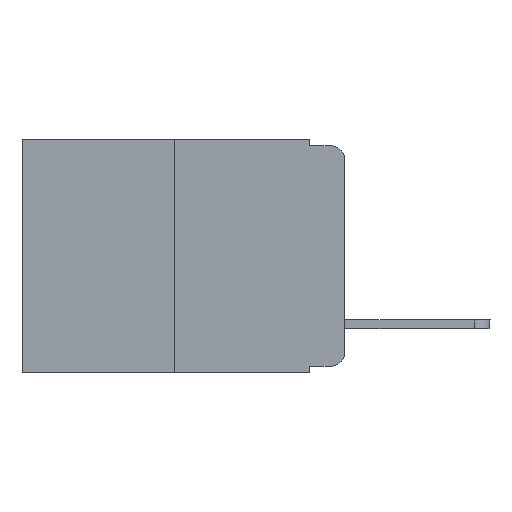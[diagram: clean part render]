
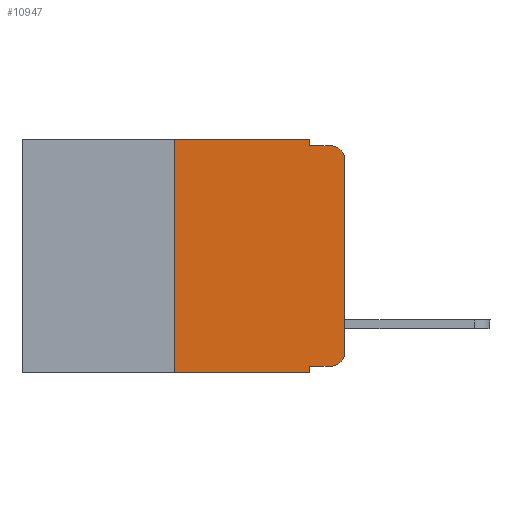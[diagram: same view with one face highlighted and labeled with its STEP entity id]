
A CAD part, left-side view. The second image highlights one B-rep face of the part: STEP entity #10947.
In plain terms, the highlighted planar face has unit normal (-1, 0, 0).
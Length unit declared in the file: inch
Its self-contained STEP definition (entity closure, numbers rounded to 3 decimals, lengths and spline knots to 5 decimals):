
#72 = FACE_OUTER_BOUND ( 'NONE', #15163, .T. ) ;
#231 = DIRECTION ( 'NONE',  ( 0., -1., 0. ) ) ;
#659 = ORIENTED_EDGE ( 'NONE', *, *, #20323, .T. ) ;
#1126 = EDGE_CURVE ( 'NONE', #13581, #15890, #11371, .T. ) ;
#1616 = ORIENTED_EDGE ( 'NONE', *, *, #21840, .T. ) ;
#1779 = VECTOR ( 'NONE', #21901, 39.37008 ) ;
#1964 = DIRECTION ( 'NONE',  ( 0., 0., -1. ) ) ;
#2164 = ORIENTED_EDGE ( 'NONE', *, *, #3324, .F. ) ;
#2433 = CARTESIAN_POINT ( 'NONE',  ( 0., 0.051, -0.333 ) ) ;
#2524 = EDGE_CURVE ( 'NONE', #21468, #22609, #14028, .T. ) ;
#2973 = CARTESIAN_POINT ( 'NONE',  ( 0., 0.02, -0.313 ) ) ;
#3324 = EDGE_CURVE ( 'NONE', #13582, #17966, #4397, .T. ) ;
#3411 = CARTESIAN_POINT ( 'NONE',  ( 0., 0.473, -0.343 ) ) ;
#3530 = ORIENTED_EDGE ( 'NONE', *, *, #21485, .F. ) ;
#4397 = LINE ( 'NONE', #21255, #16966 ) ;
#4844 = ORIENTED_EDGE ( 'NONE', *, *, #22653, .T. ) ;
#4925 = CARTESIAN_POINT ( 'NONE',  ( 0., 0.02, -0.03 ) ) ;
#5082 = DIRECTION ( 'NONE',  ( 1., 0., 0. ) ) ;
#5148 = DIRECTION ( 'NONE',  ( 0., 0., 1. ) ) ;
#5530 = CARTESIAN_POINT ( 'NONE',  ( 0., 0.051, 0. ) ) ;
#6294 = ORIENTED_EDGE ( 'NONE', *, *, #1126, .T. ) ;
#6422 = LINE ( 'NONE', #8945, #10729 ) ;
#7497 = ORIENTED_EDGE ( 'NONE', *, *, #10085, .F. ) ;
#8257 = CARTESIAN_POINT ( 'NONE',  ( 0., 0.473, 0. ) ) ;
#8421 = ORIENTED_EDGE ( 'NONE', *, *, #2524, .F. ) ;
#8534 = VECTOR ( 'NONE', #13501, 39.37008 ) ;
#8799 = LINE ( 'NONE', #11994, #12152 ) ;
#8945 = CARTESIAN_POINT ( 'NONE',  ( 0., 0., 0. ) ) ;
#9048 = DIRECTION ( 'NONE',  ( 0., 0., -1. ) ) ;
#9422 = VERTEX_POINT ( 'NONE', #17169 ) ;
#9722 = CARTESIAN_POINT ( 'NONE',  ( 0., 0.25, 0. ) ) ;
#10085 = EDGE_CURVE ( 'NONE', #22609, #16225, #21565, .T. ) ;
#10180 = CARTESIAN_POINT ( 'NONE',  ( 0., 0., -0.03 ) ) ;
#10729 = VECTOR ( 'NONE', #5148, 39.37008 ) ;
#10849 = PLANE ( 'NONE',  #12324 ) ;
#10947 = ADVANCED_FACE ( 'NONE', ( #72 ), #10849, .F. ) ;
#11371 = CIRCLE ( 'NONE', #17927, 0.02 ) ;
#11977 = VERTEX_POINT ( 'NONE', #14732 ) ;
#11994 = CARTESIAN_POINT ( 'NONE',  ( 0., 0.051, -0.01 ) ) ;
#12152 = VECTOR ( 'NONE', #231, 39.37008 ) ;
#12222 = LINE ( 'NONE', #15405, #17736 ) ;
#12324 = AXIS2_PLACEMENT_3D ( 'NONE', #18709, #5082, #9048 ) ;
#12491 = CARTESIAN_POINT ( 'NONE',  ( 0., 0.051, -0.343 ) ) ;
#13200 = CARTESIAN_POINT ( 'NONE',  ( 0., 0.02, -0.333 ) ) ;
#13342 = VECTOR ( 'NONE', #16774, 39.37008 ) ;
#13434 = LINE ( 'NONE', #3411, #8534 ) ;
#13501 = DIRECTION ( 'NONE',  ( 0., -1., 0. ) ) ;
#13581 = VERTEX_POINT ( 'NONE', #10180 ) ;
#13582 = VERTEX_POINT ( 'NONE', #2433 ) ;
#14028 = LINE ( 'NONE', #8257, #1779 ) ;
#14034 = CIRCLE ( 'NONE', #18065, 0.02 ) ;
#14286 = VECTOR ( 'NONE', #23396, 39.37008 ) ;
#14572 = CARTESIAN_POINT ( 'NONE',  ( 0., 0.051, -0.01 ) ) ;
#14732 = CARTESIAN_POINT ( 'NONE',  ( 0., 0.25, -0.343 ) ) ;
#14760 = ORIENTED_EDGE ( 'NONE', *, *, #23167, .F. ) ;
#15163 = EDGE_LOOP ( 'NONE', ( #17687, #6294, #3530, #7497, #8421, #14760, #4844, #2164, #1616, #659 ) ) ;
#15405 = CARTESIAN_POINT ( 'NONE',  ( 0., 0.051, -0.333 ) ) ;
#15815 = DIRECTION ( 'NONE',  ( -1., 0., 0. ) ) ;
#15890 = VERTEX_POINT ( 'NONE', #23428 ) ;
#16225 = VERTEX_POINT ( 'NONE', #14572 ) ;
#16395 = DIRECTION ( 'NONE',  ( 0., 0., -1. ) ) ;
#16566 = DIRECTION ( 'NONE',  ( -1., 0., 0. ) ) ;
#16774 = DIRECTION ( 'NONE',  ( 0., 0., -1. ) ) ;
#16966 = VECTOR ( 'NONE', #17351, 39.37008 ) ;
#17059 = LINE ( 'NONE', #9722, #14286 ) ;
#17169 = CARTESIAN_POINT ( 'NONE',  ( 0., 0., -0.313 ) ) ;
#17351 = DIRECTION ( 'NONE',  ( 0., 0., -1. ) ) ;
#17687 = ORIENTED_EDGE ( 'NONE', *, *, #19193, .T. ) ;
#17736 = VECTOR ( 'NONE', #21120, 39.37008 ) ;
#17927 = AXIS2_PLACEMENT_3D ( 'NONE', #4925, #15815, #1964 ) ;
#17966 = VERTEX_POINT ( 'NONE', #12491 ) ;
#17986 = CARTESIAN_POINT ( 'NONE',  ( 0., 0.25, 0. ) ) ;
#18065 = AXIS2_PLACEMENT_3D ( 'NONE', #2973, #16566, #16395 ) ;
#18709 = CARTESIAN_POINT ( 'NONE',  ( 0., 0.473, 0. ) ) ;
#18757 = CARTESIAN_POINT ( 'NONE',  ( 0., 0.051, 0. ) ) ;
#19193 = EDGE_CURVE ( 'NONE', #9422, #13581, #6422, .T. ) ;
#20323 = EDGE_CURVE ( 'NONE', #23644, #9422, #14034, .T. ) ;
#21120 = DIRECTION ( 'NONE',  ( 0., -1., 0. ) ) ;
#21255 = CARTESIAN_POINT ( 'NONE',  ( 0., 0.051, 0. ) ) ;
#21468 = VERTEX_POINT ( 'NONE', #17986 ) ;
#21485 = EDGE_CURVE ( 'NONE', #16225, #15890, #8799, .T. ) ;
#21565 = LINE ( 'NONE', #18757, #13342 ) ;
#21840 = EDGE_CURVE ( 'NONE', #13582, #23644, #12222, .T. ) ;
#21901 = DIRECTION ( 'NONE',  ( 0., -1., 0. ) ) ;
#22609 = VERTEX_POINT ( 'NONE', #5530 ) ;
#22653 = EDGE_CURVE ( 'NONE', #11977, #17966, #13434, .T. ) ;
#23167 = EDGE_CURVE ( 'NONE', #11977, #21468, #17059, .T. ) ;
#23396 = DIRECTION ( 'NONE',  ( 0., 0., 1. ) ) ;
#23428 = CARTESIAN_POINT ( 'NONE',  ( 0., 0.02, -0.01 ) ) ;
#23644 = VERTEX_POINT ( 'NONE', #13200 ) ;
